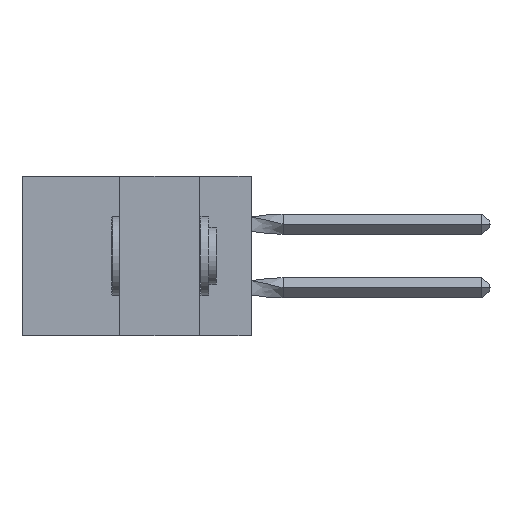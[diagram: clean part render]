
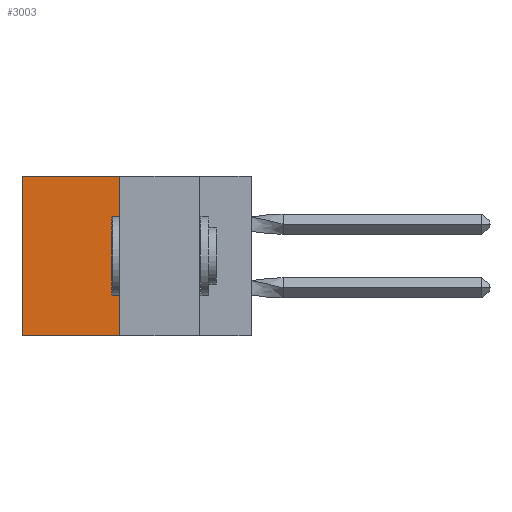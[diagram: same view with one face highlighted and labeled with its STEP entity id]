
A CAD part, left-side view. The second image highlights one B-rep face of the part: STEP entity #3003.
In plain terms, the highlighted planar face has unit normal (-1, 0, 0).
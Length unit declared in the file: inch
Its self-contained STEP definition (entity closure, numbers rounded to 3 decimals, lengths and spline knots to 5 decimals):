
#677 = PLANE ( 'NONE',  #13927 ) ;
#828 = VERTEX_POINT ( 'NONE', #6834 ) ;
#1602 = CARTESIAN_POINT ( 'NONE',  ( 0.305, 0.413, -0.5 ) ) ;
#2177 = EDGE_CURVE ( 'NONE', #828, #8156, #19682, .T. ) ;
#2363 = DIRECTION ( 'NONE',  ( 0., 0., -1. ) ) ;
#2789 = EDGE_LOOP ( 'NONE', ( #16580, #30499, #7971, #9095 ) ) ;
#3003 = ADVANCED_FACE ( 'NONE', ( #18870 ), #677, .F. ) ;
#3224 = DIRECTION ( 'NONE',  ( 0., 0., -1. ) ) ;
#4151 = EDGE_CURVE ( 'NONE', #12877, #11015, #12157, .T. ) ;
#4253 = CARTESIAN_POINT ( 'NONE',  ( 0.305, 0.72, -0.5 ) ) ;
#4576 = EDGE_CURVE ( 'NONE', #11015, #8156, #15368, .T. ) ;
#6049 = CARTESIAN_POINT ( 'NONE',  ( 0.305, 0.413, 0. ) ) ;
#6333 = DIRECTION ( 'NONE',  ( 0., 1., 0. ) ) ;
#6834 = CARTESIAN_POINT ( 'NONE',  ( 0.305, 0.72, 0. ) ) ;
#7971 = ORIENTED_EDGE ( 'NONE', *, *, #4151, .F. ) ;
#8156 = VERTEX_POINT ( 'NONE', #4253 ) ;
#9095 = ORIENTED_EDGE ( 'NONE', *, *, #23066, .T. ) ;
#9464 = VECTOR ( 'NONE', #6333, 39.37008 ) ;
#11015 = VERTEX_POINT ( 'NONE', #14096 ) ;
#11512 = VECTOR ( 'NONE', #28539, 39.37008 ) ;
#12157 = LINE ( 'NONE', #32490, #28318 ) ;
#12877 = VERTEX_POINT ( 'NONE', #14299 ) ;
#13927 = AXIS2_PLACEMENT_3D ( 'NONE', #25654, #28197, #3224 ) ;
#14096 = CARTESIAN_POINT ( 'NONE',  ( 0.305, 0.413, -0.5 ) ) ;
#14299 = CARTESIAN_POINT ( 'NONE',  ( 0.305, 0.413, 0. ) ) ;
#14730 = DIRECTION ( 'NONE',  ( 0., 0., -1. ) ) ;
#15368 = LINE ( 'NONE', #1602, #9464 ) ;
#16580 = ORIENTED_EDGE ( 'NONE', *, *, #2177, .T. ) ;
#18870 = FACE_OUTER_BOUND ( 'NONE', #2789, .T. ) ;
#19310 = VECTOR ( 'NONE', #2363, 39.37008 ) ;
#19682 = LINE ( 'NONE', #19942, #19310 ) ;
#19942 = CARTESIAN_POINT ( 'NONE',  ( 0.305, 0.72, -0.5 ) ) ;
#23066 = EDGE_CURVE ( 'NONE', #12877, #828, #29221, .T. ) ;
#25654 = CARTESIAN_POINT ( 'NONE',  ( 0.305, 0.413, -0.5 ) ) ;
#28197 = DIRECTION ( 'NONE',  ( 1., 0., 0. ) ) ;
#28318 = VECTOR ( 'NONE', #14730, 39.37008 ) ;
#28539 = DIRECTION ( 'NONE',  ( 0., 1., 0. ) ) ;
#29221 = LINE ( 'NONE', #6049, #11512 ) ;
#30499 = ORIENTED_EDGE ( 'NONE', *, *, #4576, .F. ) ;
#32490 = CARTESIAN_POINT ( 'NONE',  ( 0.305, 0.413, -0.5 ) ) ;
